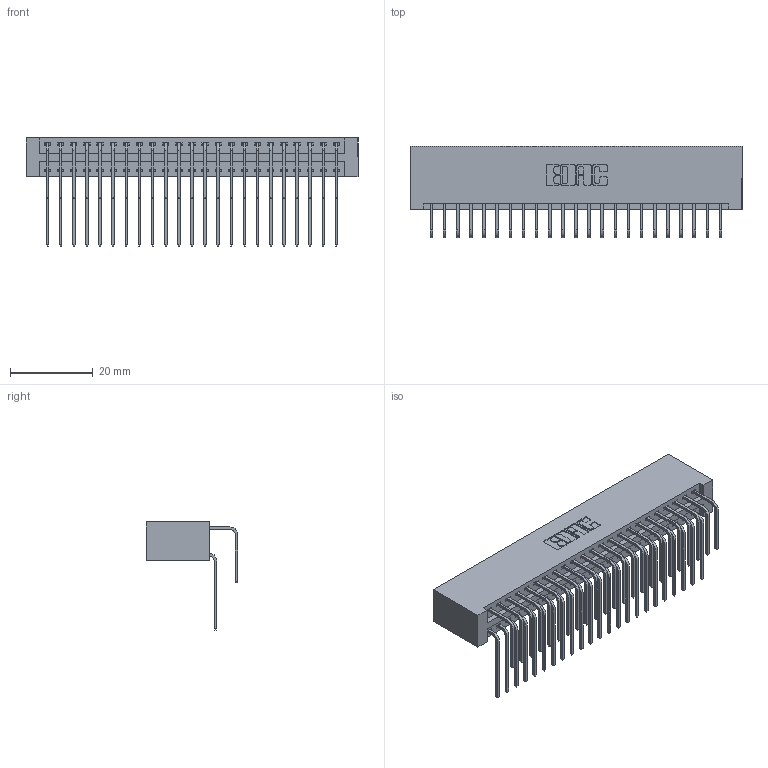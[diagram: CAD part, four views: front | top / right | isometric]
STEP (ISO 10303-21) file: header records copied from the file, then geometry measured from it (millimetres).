
FILE_DESCRIPTION (( 'STEP AP203' ), '1' );
FILE_NAME ('346-046-558-201.STEP', '2018-08-25T06:25:58', ( '' ), ( '' ), 'SwSTEP 2.0', 'SolidWorks 2016', '' );
FILE_SCHEMA (( 'CONFIG_CONTROL_DESIGN' ));
Length unit declared in the file: inch
Products named in the file (4): 346-046-558-201; 346 Part_No Mounting Lugs; 345-292-001_558 559 Tail - 1; 345-292-001_558 Tail - 2
Assembly tree (47 placements, depth 2):
  346-046-558-201
    346 Part_No Mounting Lugs
    345-292-001_558 559 Tail - 1  x23
    345-292-001_558 Tail - 2  x23
Bounding box: 80.26 x 22.16 x 26.16 mm (x, y, z)
Volume: 8517.8 mm3; surface area: 12845.9 mm2
Topology: 47 solids, 47 shells, 2598 faces, 7711 edges, 5078 vertices
Faces by surface type: plane 1774, cylinder 824
Entity records: 19075 total; most frequent: CARTESIAN_POINT 3219, ORIENTED_EDGE 3102, DIRECTION 2855, EDGE_CURVE 1551, VECTOR 1295, LINE 1295, VERTEX_POINT 1030, AXIS2_PLACEMENT_3D 780
